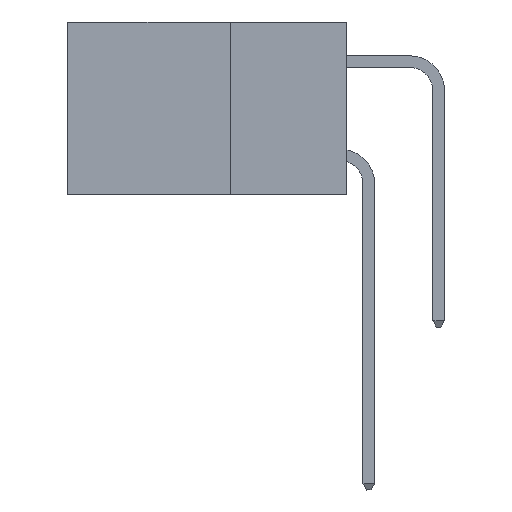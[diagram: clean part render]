
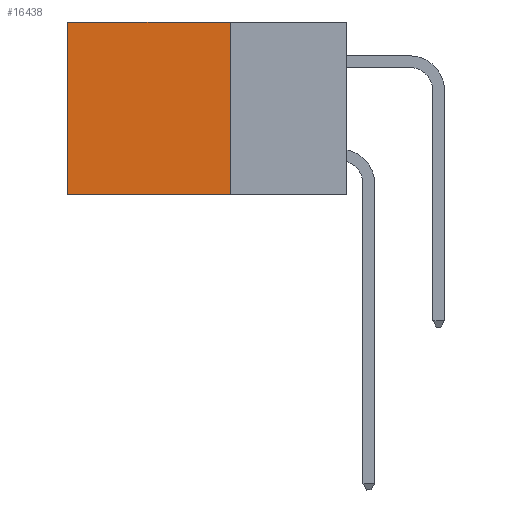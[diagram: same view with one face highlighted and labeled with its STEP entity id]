
A CAD part, left-side view. The second image highlights one B-rep face of the part: STEP entity #16438.
In plain terms, the highlighted planar face has unit normal (-1, 0, 0).
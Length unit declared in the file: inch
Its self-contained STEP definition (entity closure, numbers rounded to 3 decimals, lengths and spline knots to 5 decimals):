
#415 = VERTEX_POINT ( 'NONE', #24960 ) ;
#2026 = CARTESIAN_POINT ( 'NONE',  ( 0.2875, 0.25, 0. ) ) ;
#2436 = DIRECTION ( 'NONE',  ( 0., 1., 0. ) ) ;
#2834 = LINE ( 'NONE', #19237, #11553 ) ;
#4073 = VECTOR ( 'NONE', #28888, 39.37008 ) ;
#5983 = VERTEX_POINT ( 'NONE', #6829 ) ;
#6773 = DIRECTION ( 'NONE',  ( 0., 0., -1. ) ) ;
#6829 = CARTESIAN_POINT ( 'NONE',  ( 0.2875, 0.6, -0.37 ) ) ;
#6895 = EDGE_CURVE ( 'NONE', #415, #15765, #22280, .T. ) ;
#9049 = DIRECTION ( 'NONE',  ( 0., 1., 0. ) ) ;
#9542 = LINE ( 'NONE', #2026, #21581 ) ;
#9878 = ORIENTED_EDGE ( 'NONE', *, *, #21360, .T. ) ;
#11553 = VECTOR ( 'NONE', #2436, 39.37008 ) ;
#11717 = DIRECTION ( 'NONE',  ( 1., 0., 0. ) ) ;
#13507 = ORIENTED_EDGE ( 'NONE', *, *, #6895, .F. ) ;
#15765 = VERTEX_POINT ( 'NONE', #24496 ) ;
#16438 = ADVANCED_FACE ( 'NONE', ( #16483 ), #28320, .F. ) ;
#16483 = FACE_OUTER_BOUND ( 'NONE', #29324, .T. ) ;
#16628 = EDGE_CURVE ( 'NONE', #30132, #5983, #27932, .T. ) ;
#17156 = ORIENTED_EDGE ( 'NONE', *, *, #16628, .T. ) ;
#19237 = CARTESIAN_POINT ( 'NONE',  ( 0.2875, 0.25, -0.37 ) ) ;
#20641 = EDGE_CURVE ( 'NONE', #15765, #5983, #2834, .T. ) ;
#21360 = EDGE_CURVE ( 'NONE', #415, #30132, #9542, .T. ) ;
#21414 = DIRECTION ( 'NONE',  ( 0., 0., -1. ) ) ;
#21581 = VECTOR ( 'NONE', #9049, 39.37008 ) ;
#22280 = LINE ( 'NONE', #25969, #24920 ) ;
#23961 = ORIENTED_EDGE ( 'NONE', *, *, #20641, .F. ) ;
#24496 = CARTESIAN_POINT ( 'NONE',  ( 0.2875, 0.25, -0.37 ) ) ;
#24920 = VECTOR ( 'NONE', #6773, 39.37008 ) ;
#24960 = CARTESIAN_POINT ( 'NONE',  ( 0.2875, 0.25, 0. ) ) ;
#25969 = CARTESIAN_POINT ( 'NONE',  ( 0.2875, 0.25, 0. ) ) ;
#26873 = CARTESIAN_POINT ( 'NONE',  ( 0.2875, 0.6, 0. ) ) ;
#27932 = LINE ( 'NONE', #26873, #4073 ) ;
#28320 = PLANE ( 'NONE',  #30487 ) ;
#28888 = DIRECTION ( 'NONE',  ( 0., 0., -1. ) ) ;
#29324 = EDGE_LOOP ( 'NONE', ( #17156, #23961, #13507, #9878 ) ) ;
#30132 = VERTEX_POINT ( 'NONE', #31130 ) ;
#30487 = AXIS2_PLACEMENT_3D ( 'NONE', #30837, #11717, #21414 ) ;
#30837 = CARTESIAN_POINT ( 'NONE',  ( 0.2875, 0.25, 0. ) ) ;
#31130 = CARTESIAN_POINT ( 'NONE',  ( 0.2875, 0.6, 0. ) ) ;
